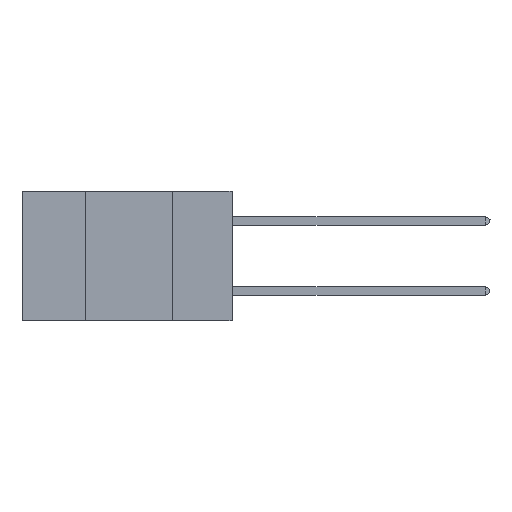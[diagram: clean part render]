
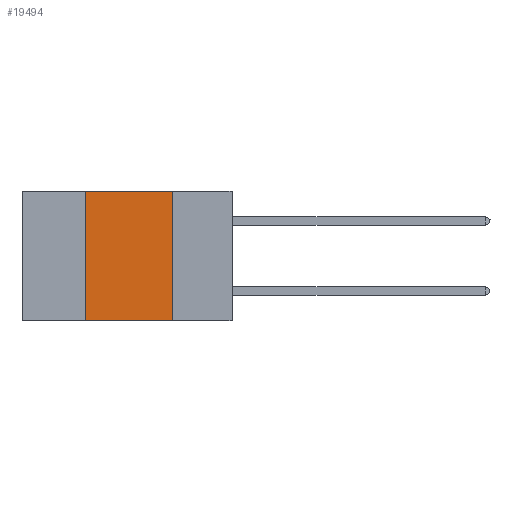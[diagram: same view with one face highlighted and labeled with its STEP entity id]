
A CAD part, left-side view. The second image highlights one B-rep face of the part: STEP entity #19494.
In plain terms, the highlighted planar face has unit normal (-1, 0, 0).
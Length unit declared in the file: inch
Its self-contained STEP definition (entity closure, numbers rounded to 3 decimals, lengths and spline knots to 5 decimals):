
#1943 = CARTESIAN_POINT ( 'NONE',  ( 0., 0.42, 0. ) ) ;
#4087 = AXIS2_PLACEMENT_3D ( 'NONE', #19903, #29905, #43753 ) ;
#7401 = EDGE_LOOP ( 'NONE', ( #40477, #15087, #39718, #25631 ) ) ;
#8325 = VERTEX_POINT ( 'NONE', #19677 ) ;
#9168 = VECTOR ( 'NONE', #22453, 39.37008 ) ;
#9709 = CARTESIAN_POINT ( 'NONE',  ( 0., 0.17, 0. ) ) ;
#12259 = DIRECTION ( 'NONE',  ( 0., -1., 0. ) ) ;
#12573 = EDGE_CURVE ( 'NONE', #31778, #8325, #43532, .T. ) ;
#13233 = PLANE ( 'NONE',  #4087 ) ;
#13375 = DIRECTION ( 'NONE',  ( 0., 0., -1. ) ) ;
#15006 = EDGE_CURVE ( 'NONE', #25040, #31778, #39648, .T. ) ;
#15087 = ORIENTED_EDGE ( 'NONE', *, *, #15006, .F. ) ;
#16552 = VERTEX_POINT ( 'NONE', #43910 ) ;
#19494 = ADVANCED_FACE ( 'NONE', ( #35227 ), #13233, .F. ) ;
#19677 = CARTESIAN_POINT ( 'NONE',  ( 0., 0.17, -0.37 ) ) ;
#19903 = CARTESIAN_POINT ( 'NONE',  ( 0., 0.6, 0. ) ) ;
#21433 = VECTOR ( 'NONE', #12259, 39.37008 ) ;
#22453 = DIRECTION ( 'NONE',  ( 0., 0., 1. ) ) ;
#22959 = LINE ( 'NONE', #1943, #9168 ) ;
#23867 = VECTOR ( 'NONE', #35038, 39.37008 ) ;
#25040 = VERTEX_POINT ( 'NONE', #31425 ) ;
#25631 = ORIENTED_EDGE ( 'NONE', *, *, #35240, .T. ) ;
#28148 = LINE ( 'NONE', #41451, #23867 ) ;
#28610 = CARTESIAN_POINT ( 'NONE',  ( 0., 0.6, 0. ) ) ;
#29438 = CARTESIAN_POINT ( 'NONE',  ( 0., 0.17, 0. ) ) ;
#29905 = DIRECTION ( 'NONE',  ( 1., 0., 0. ) ) ;
#31425 = CARTESIAN_POINT ( 'NONE',  ( 0., 0.42, 0. ) ) ;
#31778 = VERTEX_POINT ( 'NONE', #29438 ) ;
#34979 = VECTOR ( 'NONE', #13375, 39.37008 ) ;
#35038 = DIRECTION ( 'NONE',  ( 0., -1., 0. ) ) ;
#35227 = FACE_OUTER_BOUND ( 'NONE', #7401, .T. ) ;
#35240 = EDGE_CURVE ( 'NONE', #16552, #8325, #28148, .T. ) ;
#39648 = LINE ( 'NONE', #28610, #21433 ) ;
#39718 = ORIENTED_EDGE ( 'NONE', *, *, #41479, .F. ) ;
#40477 = ORIENTED_EDGE ( 'NONE', *, *, #12573, .F. ) ;
#41451 = CARTESIAN_POINT ( 'NONE',  ( 0., 0.6, -0.37 ) ) ;
#41479 = EDGE_CURVE ( 'NONE', #16552, #25040, #22959, .T. ) ;
#43532 = LINE ( 'NONE', #9709, #34979 ) ;
#43753 = DIRECTION ( 'NONE',  ( 0., 0., -1. ) ) ;
#43910 = CARTESIAN_POINT ( 'NONE',  ( 0., 0.42, -0.37 ) ) ;
